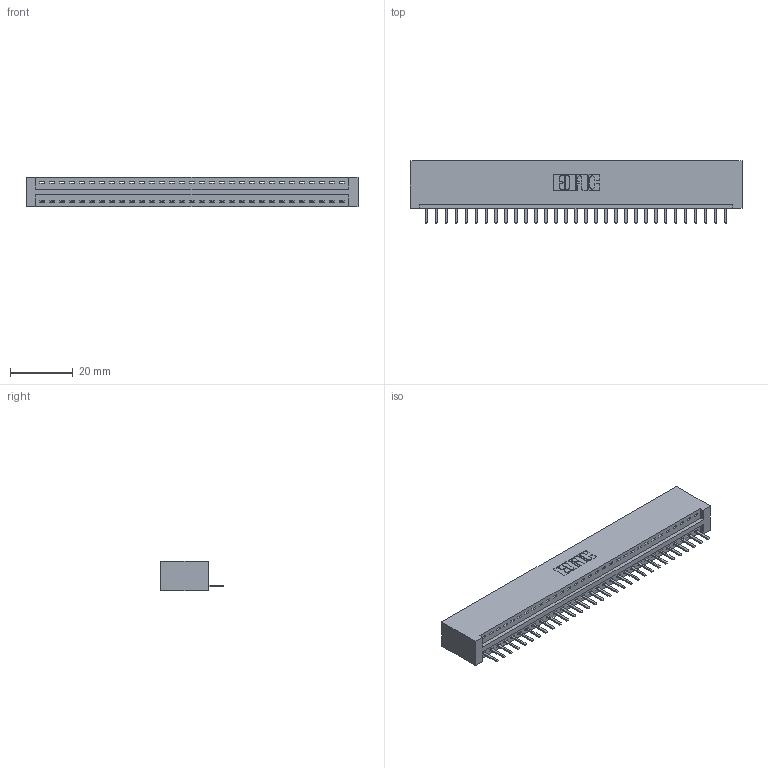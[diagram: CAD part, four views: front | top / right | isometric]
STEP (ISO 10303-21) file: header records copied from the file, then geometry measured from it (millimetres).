
FILE_DESCRIPTION (( 'STEP AP203' ), '1' );
FILE_NAME ('396-031-520-101.STEP', '2019-10-27T10:48:15', ( '' ), ( '' ), 'SwSTEP 2.0', 'SolidWorks 2016', '' );
FILE_SCHEMA (( 'CONFIG_CONTROL_DESIGN' ));
Length unit declared in the file: inch
Products named in the file (3): 346 Part_No Mounting Lugs; 396-031-520-101; 345-292-001_345-293-120
Assembly tree (32 placements, depth 2):
  396-031-520-101
    346 Part_No Mounting Lugs
    345-292-001_345-293-120  x31
Bounding box: 105.66 x 20.02 x 9.4 mm (x, y, z)
Volume: 10498.8 mm3; surface area: 12780.9 mm2
Topology: 32 solids, 32 shells, 2036 faces, 6009 edges, 3922 vertices
Faces by surface type: plane 1374, cylinder 662
Entity records: 20557 total; most frequent: CARTESIAN_POINT 3545, ORIENTED_EDGE 3498, DIRECTION 3123, EDGE_CURVE 1749, VECTOR 1497, LINE 1497, VERTEX_POINT 1162, AXIS2_PLACEMENT_3D 813
